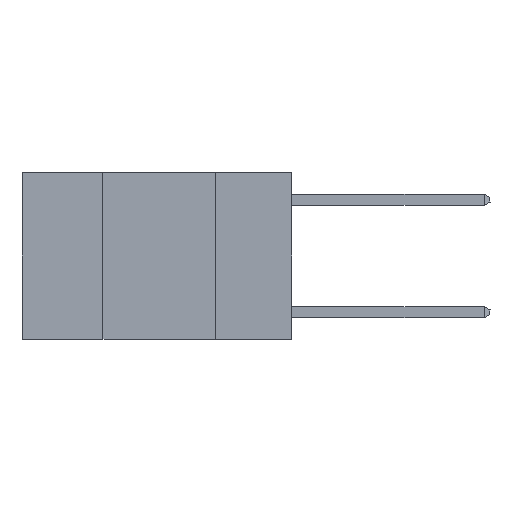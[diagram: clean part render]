
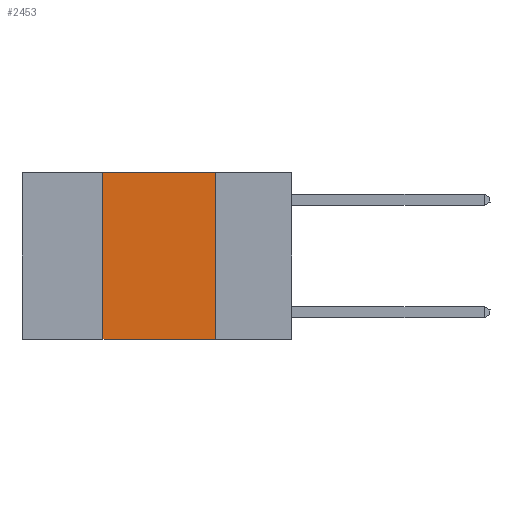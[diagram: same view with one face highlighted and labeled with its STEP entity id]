
A CAD part, left-side view. The second image highlights one B-rep face of the part: STEP entity #2453.
In plain terms, the highlighted planar face has unit normal (-1, 0, 0).
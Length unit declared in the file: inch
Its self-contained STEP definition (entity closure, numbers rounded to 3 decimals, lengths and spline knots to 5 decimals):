
#160 = EDGE_CURVE ( 'NONE', #8331, #14804, #3008, .T. ) ;
#188 = CARTESIAN_POINT ( 'NONE',  ( 0., 0.42, -0.37 ) ) ;
#287 = CARTESIAN_POINT ( 'NONE',  ( 0., 0.17, 0. ) ) ;
#458 = ORIENTED_EDGE ( 'NONE', *, *, #3550, .F. ) ;
#1739 = VERTEX_POINT ( 'NONE', #9930 ) ;
#2298 = DIRECTION ( 'NONE',  ( 0., 0., 1. ) ) ;
#2453 = ADVANCED_FACE ( 'NONE', ( #16405 ), #19335, .F. ) ;
#2586 = CARTESIAN_POINT ( 'NONE',  ( 0., 0.17, -0.37 ) ) ;
#2705 = CARTESIAN_POINT ( 'NONE',  ( 0., 0.17, 0. ) ) ;
#2930 = VECTOR ( 'NONE', #18098, 39.37008 ) ;
#3008 = LINE ( 'NONE', #16425, #17208 ) ;
#3480 = CARTESIAN_POINT ( 'NONE',  ( 0., 0.6, 0. ) ) ;
#3550 = EDGE_CURVE ( 'NONE', #10029, #14804, #3994, .T. ) ;
#3994 = LINE ( 'NONE', #2705, #2930 ) ;
#4032 = ORIENTED_EDGE ( 'NONE', *, *, #160, .T. ) ;
#5701 = CARTESIAN_POINT ( 'NONE',  ( 0., 0.42, 0. ) ) ;
#6200 = EDGE_LOOP ( 'NONE', ( #458, #21260, #18283, #4032 ) ) ;
#7008 = EDGE_CURVE ( 'NONE', #1739, #10029, #8694, .T. ) ;
#8331 = VERTEX_POINT ( 'NONE', #188 ) ;
#8694 = LINE ( 'NONE', #3480, #21077 ) ;
#9930 = CARTESIAN_POINT ( 'NONE',  ( 0., 0.42, 0. ) ) ;
#10015 = DIRECTION ( 'NONE',  ( 0., -1., 0. ) ) ;
#10029 = VERTEX_POINT ( 'NONE', #287 ) ;
#11255 = LINE ( 'NONE', #5701, #15756 ) ;
#13033 = DIRECTION ( 'NONE',  ( 1., 0., 0. ) ) ;
#14226 = CARTESIAN_POINT ( 'NONE',  ( 0., 0.6, 0. ) ) ;
#14804 = VERTEX_POINT ( 'NONE', #2586 ) ;
#15756 = VECTOR ( 'NONE', #2298, 39.37008 ) ;
#16405 = FACE_OUTER_BOUND ( 'NONE', #6200, .T. ) ;
#16425 = CARTESIAN_POINT ( 'NONE',  ( 0., 0.6, -0.37 ) ) ;
#17208 = VECTOR ( 'NONE', #10015, 39.37008 ) ;
#18098 = DIRECTION ( 'NONE',  ( 0., 0., -1. ) ) ;
#18283 = ORIENTED_EDGE ( 'NONE', *, *, #20809, .F. ) ;
#18497 = AXIS2_PLACEMENT_3D ( 'NONE', #14226, #13033, #19061 ) ;
#18798 = DIRECTION ( 'NONE',  ( 0., -1., 0. ) ) ;
#19061 = DIRECTION ( 'NONE',  ( 0., 0., -1. ) ) ;
#19335 = PLANE ( 'NONE',  #18497 ) ;
#20809 = EDGE_CURVE ( 'NONE', #8331, #1739, #11255, .T. ) ;
#21077 = VECTOR ( 'NONE', #18798, 39.37008 ) ;
#21260 = ORIENTED_EDGE ( 'NONE', *, *, #7008, .F. ) ;
